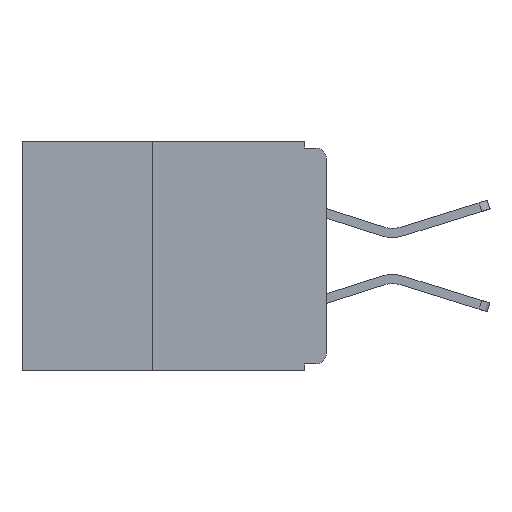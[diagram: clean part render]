
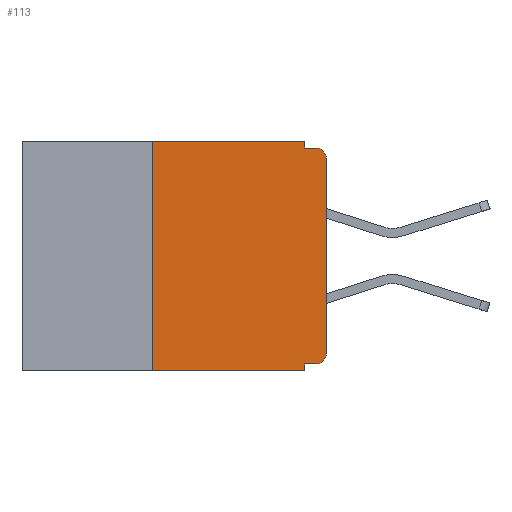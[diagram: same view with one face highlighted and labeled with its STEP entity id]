
A CAD part, left-side view. The second image highlights one B-rep face of the part: STEP entity #113.
In plain terms, the highlighted planar face has unit normal (-1, 0, 0).
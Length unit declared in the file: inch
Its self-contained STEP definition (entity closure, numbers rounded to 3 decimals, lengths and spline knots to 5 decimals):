
#38 = ORIENTED_EDGE ( 'NONE', *, *, #3798, .T. ) ;
#106 = LINE ( 'NONE', #15442, #3100 ) ;
#113 = ADVANCED_FACE ( 'NONE', ( #5728 ), #2000, .F. ) ;
#157 = EDGE_CURVE ( 'NONE', #7660, #12577, #1569, .T. ) ;
#278 = DIRECTION ( 'NONE',  ( 0., 0., 1. ) ) ;
#488 = CARTESIAN_POINT ( 'NONE',  ( 0., 0.015, -0.025 ) ) ;
#577 = CIRCLE ( 'NONE', #833, 0.015 ) ;
#702 = CARTESIAN_POINT ( 'NONE',  ( 0., 0.437, 0. ) ) ;
#808 = DIRECTION ( 'NONE',  ( 0., -1., 0. ) ) ;
#833 = AXIS2_PLACEMENT_3D ( 'NONE', #488, #9203, #1762 ) ;
#1162 = VECTOR ( 'NONE', #8216, 39.37008 ) ;
#1569 = LINE ( 'NONE', #14005, #1162 ) ;
#1762 = DIRECTION ( 'NONE',  ( 0., 0., -1. ) ) ;
#1822 = EDGE_CURVE ( 'NONE', #6911, #7855, #106, .T. ) ;
#2000 = PLANE ( 'NONE',  #8161 ) ;
#2164 = CARTESIAN_POINT ( 'NONE',  ( 0., 0.031, -0.33 ) ) ;
#2355 = AXIS2_PLACEMENT_3D ( 'NONE', #14122, #6921, #15281 ) ;
#2406 = ORIENTED_EDGE ( 'NONE', *, *, #6708, .F. ) ;
#2505 = VERTEX_POINT ( 'NONE', #9286 ) ;
#2545 = CARTESIAN_POINT ( 'NONE',  ( 0., 0.015, -0.32 ) ) ;
#2611 = ORIENTED_EDGE ( 'NONE', *, *, #5626, .F. ) ;
#2620 = CARTESIAN_POINT ( 'NONE',  ( 0., 0.031, -0.01 ) ) ;
#3100 = VECTOR ( 'NONE', #4545, 39.37008 ) ;
#3527 = ORIENTED_EDGE ( 'NONE', *, *, #14874, .F. ) ;
#3672 = LINE ( 'NONE', #5300, #6959 ) ;
#3798 = EDGE_CURVE ( 'NONE', #13236, #5980, #6597, .T. ) ;
#3826 = VECTOR ( 'NONE', #6352, 39.37008 ) ;
#3849 = CARTESIAN_POINT ( 'NONE',  ( 0., 0., -0.305 ) ) ;
#4263 = CARTESIAN_POINT ( 'NONE',  ( 0., 0.25, -0.33 ) ) ;
#4281 = CARTESIAN_POINT ( 'NONE',  ( 0., 0.031, -0.32 ) ) ;
#4386 = ORIENTED_EDGE ( 'NONE', *, *, #157, .F. ) ;
#4545 = DIRECTION ( 'NONE',  ( 0., -1., 0. ) ) ;
#4638 = ORIENTED_EDGE ( 'NONE', *, *, #8539, .T. ) ;
#4854 = ORIENTED_EDGE ( 'NONE', *, *, #8142, .T. ) ;
#5300 = CARTESIAN_POINT ( 'NONE',  ( 0., 0.031, 0. ) ) ;
#5564 = VERTEX_POINT ( 'NONE', #2620 ) ;
#5626 = EDGE_CURVE ( 'NONE', #7855, #5564, #3672, .T. ) ;
#5648 = CARTESIAN_POINT ( 'NONE',  ( 0., 0.437, -0.33 ) ) ;
#5728 = FACE_OUTER_BOUND ( 'NONE', #6325, .T. ) ;
#5980 = VERTEX_POINT ( 'NONE', #8507 ) ;
#5991 = VERTEX_POINT ( 'NONE', #14487 ) ;
#6128 = VECTOR ( 'NONE', #15557, 39.37008 ) ;
#6325 = EDGE_LOOP ( 'NONE', ( #4854, #4638, #2406, #2611, #9917, #3527, #38, #8809, #4386, #10248 ) ) ;
#6352 = DIRECTION ( 'NONE',  ( 0., -1., 0. ) ) ;
#6597 = LINE ( 'NONE', #5648, #9424 ) ;
#6708 = EDGE_CURVE ( 'NONE', #5564, #5991, #13504, .T. ) ;
#6911 = VERTEX_POINT ( 'NONE', #8518 ) ;
#6921 = DIRECTION ( 'NONE',  ( -1., 0., 0. ) ) ;
#6959 = VECTOR ( 'NONE', #12496, 39.37008 ) ;
#6972 = VECTOR ( 'NONE', #8376, 39.37008 ) ;
#7085 = VERTEX_POINT ( 'NONE', #3849 ) ;
#7316 = DIRECTION ( 'NONE',  ( 0., 0., -1. ) ) ;
#7660 = VERTEX_POINT ( 'NONE', #2545 ) ;
#7720 = DIRECTION ( 'NONE',  ( 1., 0., 0. ) ) ;
#7855 = VERTEX_POINT ( 'NONE', #11483 ) ;
#8142 = EDGE_CURVE ( 'NONE', #7085, #2505, #15684, .T. ) ;
#8161 = AXIS2_PLACEMENT_3D ( 'NONE', #702, #7720, #7316 ) ;
#8216 = DIRECTION ( 'NONE',  ( 0., 1., 0. ) ) ;
#8376 = DIRECTION ( 'NONE',  ( 0., 0., -1. ) ) ;
#8507 = CARTESIAN_POINT ( 'NONE',  ( 0., 0.031, -0.33 ) ) ;
#8518 = CARTESIAN_POINT ( 'NONE',  ( 0., 0.25, 0. ) ) ;
#8527 = CIRCLE ( 'NONE', #2355, 0.015 ) ;
#8539 = EDGE_CURVE ( 'NONE', #2505, #5991, #577, .T. ) ;
#8809 = ORIENTED_EDGE ( 'NONE', *, *, #13450, .F. ) ;
#9203 = DIRECTION ( 'NONE',  ( -1., 0., 0. ) ) ;
#9286 = CARTESIAN_POINT ( 'NONE',  ( 0., 0., -0.025 ) ) ;
#9424 = VECTOR ( 'NONE', #808, 39.37008 ) ;
#9917 = ORIENTED_EDGE ( 'NONE', *, *, #1822, .F. ) ;
#10196 = LINE ( 'NONE', #2164, #6972 ) ;
#10248 = ORIENTED_EDGE ( 'NONE', *, *, #10339, .T. ) ;
#10339 = EDGE_CURVE ( 'NONE', #7660, #7085, #8527, .T. ) ;
#10532 = LINE ( 'NONE', #14969, #13740 ) ;
#11483 = CARTESIAN_POINT ( 'NONE',  ( 0., 0.031, 0. ) ) ;
#12355 = CARTESIAN_POINT ( 'NONE',  ( 0., 0., -0.01 ) ) ;
#12496 = DIRECTION ( 'NONE',  ( 0., 0., -1. ) ) ;
#12577 = VERTEX_POINT ( 'NONE', #4281 ) ;
#13236 = VERTEX_POINT ( 'NONE', #4263 ) ;
#13450 = EDGE_CURVE ( 'NONE', #12577, #5980, #10196, .T. ) ;
#13504 = LINE ( 'NONE', #12355, #3826 ) ;
#13740 = VECTOR ( 'NONE', #278, 39.37008 ) ;
#14005 = CARTESIAN_POINT ( 'NONE',  ( 0., 0., -0.32 ) ) ;
#14122 = CARTESIAN_POINT ( 'NONE',  ( 0., 0.015, -0.305 ) ) ;
#14407 = CARTESIAN_POINT ( 'NONE',  ( 0., 0., 0. ) ) ;
#14487 = CARTESIAN_POINT ( 'NONE',  ( 0., 0.015, -0.01 ) ) ;
#14874 = EDGE_CURVE ( 'NONE', #13236, #6911, #10532, .T. ) ;
#14969 = CARTESIAN_POINT ( 'NONE',  ( 0., 0.25, -0.33 ) ) ;
#15281 = DIRECTION ( 'NONE',  ( 0., 0., -1. ) ) ;
#15442 = CARTESIAN_POINT ( 'NONE',  ( 0., 0.437, 0. ) ) ;
#15557 = DIRECTION ( 'NONE',  ( 0., 0., 1. ) ) ;
#15684 = LINE ( 'NONE', #14407, #6128 ) ;
